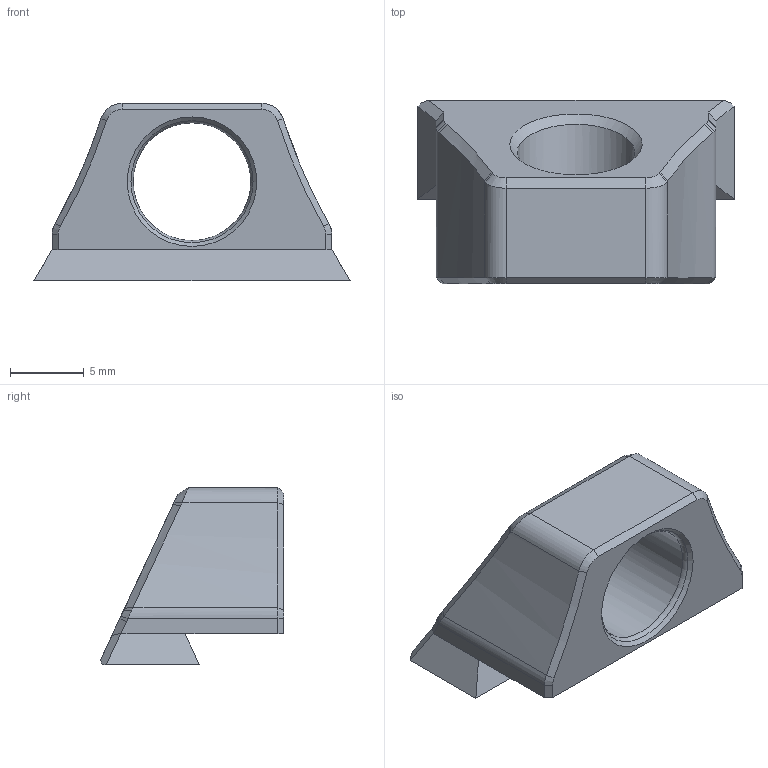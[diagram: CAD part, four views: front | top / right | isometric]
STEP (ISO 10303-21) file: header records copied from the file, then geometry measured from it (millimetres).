
FILE_DESCRIPTION(/* description */ (''),/* implementation_level */ '2;1');
FILE_NAME(/* name */ 'Ghost Ring 6.5 Rear Sight.step',/* time_stamp */ '2021-03-12T12:37:42-05:00',/* author */ (''),/* organization */ (''),/* preprocessor_version */ 'ST-DEVELOPER v18.1',/* originating_system */ 'Autodesk Translation Framework v9.10.0.1330',/* authorisation */ '');
FILE_SCHEMA (('AUTOMOTIVE_DESIGN { 1 0 10303 214 3 1 1 }'));
Length unit declared in the file: millimetre
Products named in the file (1): Ghost Ring 6.5 Rear Sight
Bounding box: 21.5 x 12.47 x 12.04 mm (x, y, z)
Volume: 1226 mm3; surface area: 1093.7 mm2
Topology: 1 solids, 1 shells, 47 faces, 117 edges, 72 vertices
Faces by surface type: plane 19, bspline 13, cone 7, cylinder 7, torus 1
Full cylindrical faces by diameter (mm): 8 x1
Entity records: 1652 total; most frequent: CARTESIAN_POINT 573, ORIENTED_EDGE 234, DIRECTION 178, EDGE_CURVE 117, LINE 72, VECTOR 72, VERTEX_POINT 72, AXIS2_PLACEMENT_3D 53
